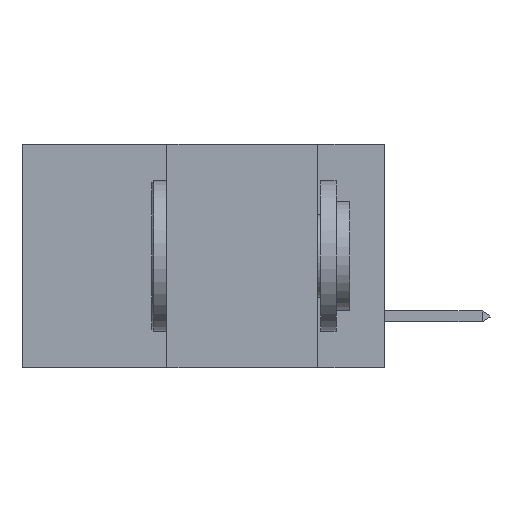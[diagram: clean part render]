
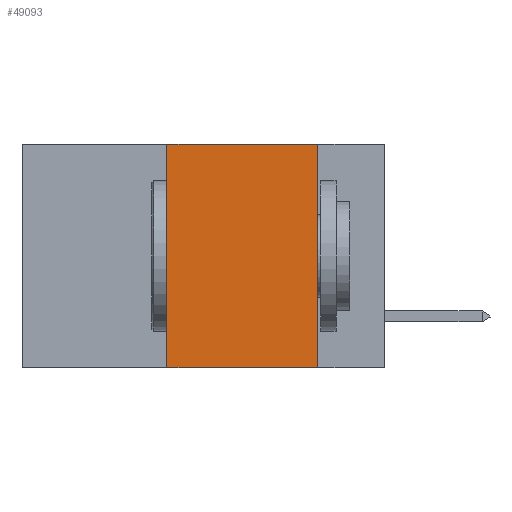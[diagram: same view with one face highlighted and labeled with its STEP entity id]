
A CAD part, left-side view. The second image highlights one B-rep face of the part: STEP entity #49093.
In plain terms, the highlighted planar face has unit normal (-1, 0, 0).
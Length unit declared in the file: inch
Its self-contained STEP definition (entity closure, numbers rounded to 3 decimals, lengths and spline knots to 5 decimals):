
#8006 = EDGE_LOOP ( 'NONE', ( #31774, #32159, #27303, #14967 ) ) ;
#10430 = DIRECTION ( 'NONE',  ( 1., 0., 0. ) ) ;
#10656 = LINE ( 'NONE', #36388, #26525 ) ;
#10801 = DIRECTION ( 'NONE',  ( 0., 0., -1. ) ) ;
#14177 = EDGE_CURVE ( 'NONE', #15978, #28229, #17753, .T. ) ;
#14189 = VERTEX_POINT ( 'NONE', #30606 ) ;
#14967 = ORIENTED_EDGE ( 'NONE', *, *, #14177, .T. ) ;
#15657 = CARTESIAN_POINT ( 'NONE',  ( 0., 0.6, 0. ) ) ;
#15978 = VERTEX_POINT ( 'NONE', #33956 ) ;
#17753 = LINE ( 'NONE', #45751, #26958 ) ;
#19005 = AXIS2_PLACEMENT_3D ( 'NONE', #34020, #10430, #10801 ) ;
#20673 = EDGE_CURVE ( 'NONE', #42289, #28229, #10656, .T. ) ;
#21479 = DIRECTION ( 'NONE',  ( 0., 0., 1. ) ) ;
#23367 = DIRECTION ( 'NONE',  ( 0., -1., 0. ) ) ;
#25628 = VECTOR ( 'NONE', #21479, 39.37008 ) ;
#26525 = VECTOR ( 'NONE', #44481, 39.37008 ) ;
#26958 = VECTOR ( 'NONE', #37503, 39.37008 ) ;
#27303 = ORIENTED_EDGE ( 'NONE', *, *, #43048, .F. ) ;
#28229 = VERTEX_POINT ( 'NONE', #36642 ) ;
#30606 = CARTESIAN_POINT ( 'NONE',  ( 0., 0.36, 0. ) ) ;
#31774 = ORIENTED_EDGE ( 'NONE', *, *, #20673, .F. ) ;
#32159 = ORIENTED_EDGE ( 'NONE', *, *, #47983, .F. ) ;
#32646 = LINE ( 'NONE', #15657, #46673 ) ;
#33852 = CARTESIAN_POINT ( 'NONE',  ( 0., 0.36, 0. ) ) ;
#33956 = CARTESIAN_POINT ( 'NONE',  ( 0., 0.36, -0.37 ) ) ;
#34020 = CARTESIAN_POINT ( 'NONE',  ( 0., 0.6, 0. ) ) ;
#35595 = FACE_OUTER_BOUND ( 'NONE', #8006, .T. ) ;
#36388 = CARTESIAN_POINT ( 'NONE',  ( 0., 0.11, 0. ) ) ;
#36642 = CARTESIAN_POINT ( 'NONE',  ( 0., 0.11, -0.37 ) ) ;
#37503 = DIRECTION ( 'NONE',  ( 0., -1., 0. ) ) ;
#40145 = LINE ( 'NONE', #33852, #25628 ) ;
#42289 = VERTEX_POINT ( 'NONE', #43763 ) ;
#43048 = EDGE_CURVE ( 'NONE', #15978, #14189, #40145, .T. ) ;
#43763 = CARTESIAN_POINT ( 'NONE',  ( 0., 0.11, 0. ) ) ;
#44481 = DIRECTION ( 'NONE',  ( 0., 0., -1. ) ) ;
#45134 = PLANE ( 'NONE',  #19005 ) ;
#45751 = CARTESIAN_POINT ( 'NONE',  ( 0., 0.6, -0.37 ) ) ;
#46673 = VECTOR ( 'NONE', #23367, 39.37008 ) ;
#47983 = EDGE_CURVE ( 'NONE', #14189, #42289, #32646, .T. ) ;
#49093 = ADVANCED_FACE ( 'NONE', ( #35595 ), #45134, .F. ) ;
